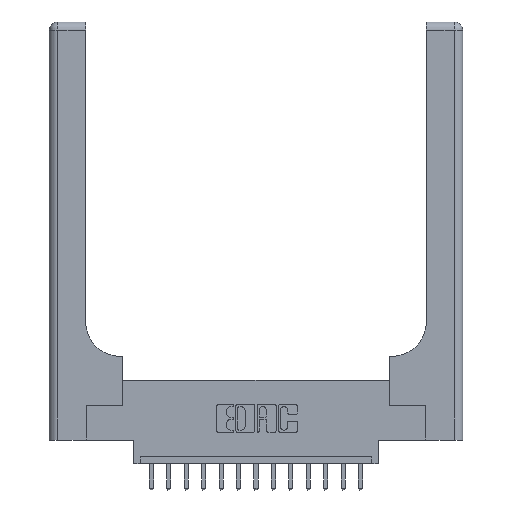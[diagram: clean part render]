
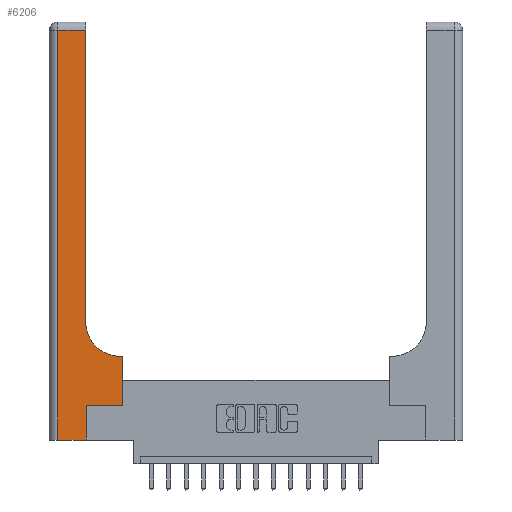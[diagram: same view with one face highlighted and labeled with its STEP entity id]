
A CAD part, top view. The second image highlights one B-rep face of the part: STEP entity #6206.
In plain terms, the highlighted planar face has unit normal (0, 0, 1).
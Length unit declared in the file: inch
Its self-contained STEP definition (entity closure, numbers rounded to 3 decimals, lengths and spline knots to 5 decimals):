
#823 = EDGE_CURVE ( 'NONE', #15489, #11270, #17171, .T. ) ;
#1395 = CARTESIAN_POINT ( 'NONE',  ( 0.265, 0.25, 0.37 ) ) ;
#1930 = LINE ( 'NONE', #3475, #10638 ) ;
#1971 = DIRECTION ( 'NONE',  ( -1., 0., 0. ) ) ;
#2129 = PLANE ( 'NONE',  #11030 ) ;
#2553 = ORIENTED_EDGE ( 'NONE', *, *, #10269, .T. ) ;
#2610 = VERTEX_POINT ( 'NONE', #9944 ) ;
#2892 = ORIENTED_EDGE ( 'NONE', *, *, #9802, .T. ) ;
#3318 = LINE ( 'NONE', #7238, #13218 ) ;
#3475 = CARTESIAN_POINT ( 'NONE',  ( 0.06, 3., 0.37 ) ) ;
#3955 = ORIENTED_EDGE ( 'NONE', *, *, #14116, .T. ) ;
#4100 = DIRECTION ( 'NONE',  ( 0., -1., 0. ) ) ;
#4341 = ORIENTED_EDGE ( 'NONE', *, *, #823, .T. ) ;
#4989 = CARTESIAN_POINT ( 'NONE',  ( 0.51, 0.85, 0.37 ) ) ;
#5140 = ORIENTED_EDGE ( 'NONE', *, *, #16225, .T. ) ;
#5306 = ORIENTED_EDGE ( 'NONE', *, *, #7626, .T. ) ;
#5728 = DIRECTION ( 'NONE',  ( -1., 0., 0. ) ) ;
#5751 = LINE ( 'NONE', #13045, #16645 ) ;
#5906 = CARTESIAN_POINT ( 'NONE',  ( 0.26, 0.6, 0.37 ) ) ;
#5968 = VECTOR ( 'NONE', #11091, 39.37008 ) ;
#5969 = DIRECTION ( 'NONE',  ( 0., 1., 0. ) ) ;
#6155 = CARTESIAN_POINT ( 'NONE',  ( 0., 3., 0.37 ) ) ;
#6158 = CARTESIAN_POINT ( 'NONE',  ( 0.06, 2.94, 0.37 ) ) ;
#6206 = ADVANCED_FACE ( 'NONE', ( #11580 ), #2129, .F. ) ;
#6377 = DIRECTION ( 'NONE',  ( 1., 0., 0. ) ) ;
#6631 = EDGE_CURVE ( 'NONE', #15248, #8886, #1930, .T. ) ;
#6917 = ORIENTED_EDGE ( 'NONE', *, *, #6631, .T. ) ;
#7163 = VERTEX_POINT ( 'NONE', #13556 ) ;
#7238 = CARTESIAN_POINT ( 'NONE',  ( 0.265, 0., 0.37 ) ) ;
#7375 = ORIENTED_EDGE ( 'NONE', *, *, #10180, .T. ) ;
#7626 = EDGE_CURVE ( 'NONE', #15653, #7163, #7850, .T. ) ;
#7850 = LINE ( 'NONE', #5906, #10815 ) ;
#8886 = VERTEX_POINT ( 'NONE', #13818 ) ;
#9034 = CARTESIAN_POINT ( 'NONE',  ( 0.26, 2.94, 0.37 ) ) ;
#9119 = CIRCLE ( 'NONE', #15493, 0.25 ) ;
#9285 = VECTOR ( 'NONE', #12143, 39.37008 ) ;
#9428 = VECTOR ( 'NONE', #15007, 39.37008 ) ;
#9802 = EDGE_CURVE ( 'NONE', #14912, #14815, #15797, .T. ) ;
#9944 = CARTESIAN_POINT ( 'NONE',  ( 0.265, 0., 0.37 ) ) ;
#10180 = EDGE_CURVE ( 'NONE', #8886, #2610, #5751, .T. ) ;
#10269 = EDGE_CURVE ( 'NONE', #7163, #15489, #9119, .T. ) ;
#10456 = ORIENTED_EDGE ( 'NONE', *, *, #13530, .T. ) ;
#10638 = VECTOR ( 'NONE', #4100, 39.37008 ) ;
#10791 = DIRECTION ( 'NONE',  ( 1., 0., 0. ) ) ;
#10815 = VECTOR ( 'NONE', #5728, 39.37008 ) ;
#11030 = AXIS2_PLACEMENT_3D ( 'NONE', #6155, #13022, #1971 ) ;
#11091 = DIRECTION ( 'NONE',  ( -1., 0., 0. ) ) ;
#11239 = CARTESIAN_POINT ( 'NONE',  ( 0.528, 0.25, 0.37 ) ) ;
#11270 = VERTEX_POINT ( 'NONE', #9034 ) ;
#11580 = FACE_OUTER_BOUND ( 'NONE', #14183, .T. ) ;
#11849 = CARTESIAN_POINT ( 'NONE',  ( 0.26, 0.85, 0.37 ) ) ;
#11923 = CARTESIAN_POINT ( 'NONE',  ( 0.528, 0.25, 0.37 ) ) ;
#12081 = LINE ( 'NONE', #13577, #5968 ) ;
#12141 = CARTESIAN_POINT ( 'NONE',  ( 0.528, 0.6, 0.37 ) ) ;
#12143 = DIRECTION ( 'NONE',  ( 0., 1., 0. ) ) ;
#12301 = VECTOR ( 'NONE', #10791, 39.37008 ) ;
#13022 = DIRECTION ( 'NONE',  ( 0., 0., -1. ) ) ;
#13045 = CARTESIAN_POINT ( 'NONE',  ( 0., 0., 0.37 ) ) ;
#13218 = VECTOR ( 'NONE', #5969, 39.37008 ) ;
#13420 = CARTESIAN_POINT ( 'NONE',  ( 0.26, 3., 0.37 ) ) ;
#13530 = EDGE_CURVE ( 'NONE', #2610, #14912, #3318, .T. ) ;
#13556 = CARTESIAN_POINT ( 'NONE',  ( 0.51, 0.6, 0.37 ) ) ;
#13577 = CARTESIAN_POINT ( 'NONE',  ( 0., 2.94, 0.37 ) ) ;
#13818 = CARTESIAN_POINT ( 'NONE',  ( 0.06, 0., 0.37 ) ) ;
#14116 = EDGE_CURVE ( 'NONE', #14815, #15653, #15880, .T. ) ;
#14183 = EDGE_LOOP ( 'NONE', ( #4341, #5140, #6917, #7375, #10456, #2892, #3955, #5306, #2553 ) ) ;
#14365 = DIRECTION ( 'NONE',  ( 1., 0., 0. ) ) ;
#14382 = DIRECTION ( 'NONE',  ( 0., 0., -1. ) ) ;
#14815 = VERTEX_POINT ( 'NONE', #11923 ) ;
#14912 = VERTEX_POINT ( 'NONE', #14964 ) ;
#14964 = CARTESIAN_POINT ( 'NONE',  ( 0.265, 0.25, 0.37 ) ) ;
#15007 = DIRECTION ( 'NONE',  ( 0., 1., 0. ) ) ;
#15248 = VERTEX_POINT ( 'NONE', #6158 ) ;
#15489 = VERTEX_POINT ( 'NONE', #11849 ) ;
#15493 = AXIS2_PLACEMENT_3D ( 'NONE', #4989, #14382, #6377 ) ;
#15653 = VERTEX_POINT ( 'NONE', #12141 ) ;
#15797 = LINE ( 'NONE', #1395, #12301 ) ;
#15880 = LINE ( 'NONE', #11239, #9428 ) ;
#16225 = EDGE_CURVE ( 'NONE', #11270, #15248, #12081, .T. ) ;
#16645 = VECTOR ( 'NONE', #14365, 39.37008 ) ;
#17171 = LINE ( 'NONE', #13420, #9285 ) ;
